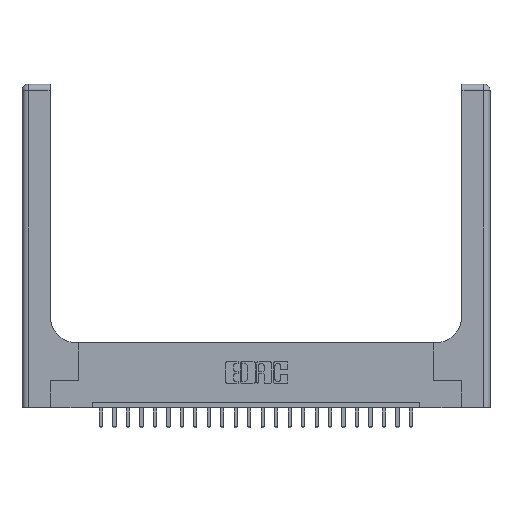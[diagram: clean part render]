
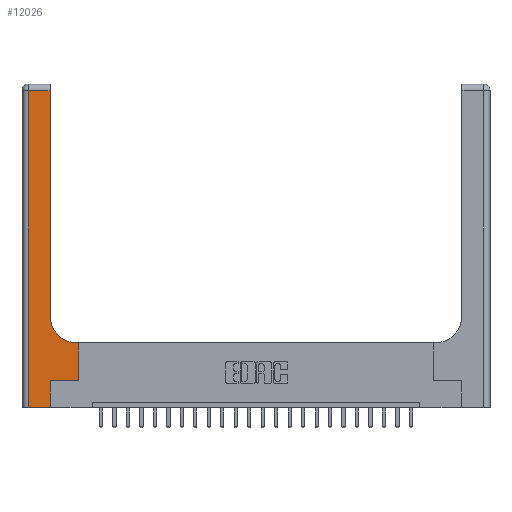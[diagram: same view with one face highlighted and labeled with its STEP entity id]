
A CAD part, top view. The second image highlights one B-rep face of the part: STEP entity #12026.
In plain terms, the highlighted planar face has unit normal (0, 0, 1).
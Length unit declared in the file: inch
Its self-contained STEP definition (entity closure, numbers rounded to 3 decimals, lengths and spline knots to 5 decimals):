
#301 = CARTESIAN_POINT ( 'NONE',  ( 0.528, 0.6, 0.37 ) ) ;
#339 = LINE ( 'NONE', #14077, #1956 ) ;
#576 = DIRECTION ( 'NONE',  ( 1., 0., 0. ) ) ;
#1641 = VECTOR ( 'NONE', #16301, 39.37008 ) ;
#1911 = CARTESIAN_POINT ( 'NONE',  ( 0.26, 3., 0.37 ) ) ;
#1956 = VECTOR ( 'NONE', #22181, 39.37008 ) ;
#2137 = ORIENTED_EDGE ( 'NONE', *, *, #9708, .T. ) ;
#2504 = EDGE_CURVE ( 'NONE', #5481, #12135, #12380, .T. ) ;
#2639 = DIRECTION ( 'NONE',  ( 1., 0., 0. ) ) ;
#2939 = CARTESIAN_POINT ( 'NONE',  ( 0.265, 0., 0.37 ) ) ;
#3023 = LINE ( 'NONE', #12256, #21039 ) ;
#3322 = ORIENTED_EDGE ( 'NONE', *, *, #9574, .T. ) ;
#3435 = CARTESIAN_POINT ( 'NONE',  ( 0.06, 3., 0.37 ) ) ;
#3584 = ORIENTED_EDGE ( 'NONE', *, *, #2504, .T. ) ;
#3600 = EDGE_CURVE ( 'NONE', #12812, #16042, #7360, .T. ) ;
#3667 = DIRECTION ( 'NONE',  ( 0., -1., 0. ) ) ;
#3821 = CARTESIAN_POINT ( 'NONE',  ( 0.06, 2.94, 0.37 ) ) ;
#3824 = FACE_OUTER_BOUND ( 'NONE', #8915, .T. ) ;
#4841 = ORIENTED_EDGE ( 'NONE', *, *, #3600, .T. ) ;
#5481 = VERTEX_POINT ( 'NONE', #21734 ) ;
#5776 = VECTOR ( 'NONE', #576, 39.37008 ) ;
#6133 = CIRCLE ( 'NONE', #20960, 0.25 ) ;
#7071 = CARTESIAN_POINT ( 'NONE',  ( 0.51, 0.6, 0.37 ) ) ;
#7234 = CARTESIAN_POINT ( 'NONE',  ( 0.26, 0.85, 0.37 ) ) ;
#7360 = LINE ( 'NONE', #17850, #18804 ) ;
#7581 = EDGE_CURVE ( 'NONE', #16042, #15617, #339, .T. ) ;
#7746 = VECTOR ( 'NONE', #2639, 39.37008 ) ;
#8087 = PLANE ( 'NONE',  #21438 ) ;
#8350 = CARTESIAN_POINT ( 'NONE',  ( 0.26, 2.94, 0.37 ) ) ;
#8547 = CARTESIAN_POINT ( 'NONE',  ( 0.265, 0.25, 0.37 ) ) ;
#8595 = VECTOR ( 'NONE', #14398, 39.37008 ) ;
#8769 = DIRECTION ( 'NONE',  ( 0., 0., -1. ) ) ;
#8854 = DIRECTION ( 'NONE',  ( 1., 0., 0. ) ) ;
#8915 = EDGE_LOOP ( 'NONE', ( #14490, #12352, #15742, #3584, #2137, #14130, #4841, #22571, #3322 ) ) ;
#9363 = DIRECTION ( 'NONE',  ( 0., 1., 0. ) ) ;
#9574 = EDGE_CURVE ( 'NONE', #15617, #15629, #6133, .T. ) ;
#9708 = EDGE_CURVE ( 'NONE', #12135, #17680, #10790, .T. ) ;
#10790 = LINE ( 'NONE', #17848, #8595 ) ;
#10931 = CARTESIAN_POINT ( 'NONE',  ( 0., 0., 0.37 ) ) ;
#10977 = LINE ( 'NONE', #1911, #1641 ) ;
#12026 = ADVANCED_FACE ( 'NONE', ( #3824 ), #8087, .F. ) ;
#12104 = CARTESIAN_POINT ( 'NONE',  ( 0.528, 0.25, 0.37 ) ) ;
#12135 = VERTEX_POINT ( 'NONE', #2939 ) ;
#12251 = VECTOR ( 'NONE', #3667, 39.37008 ) ;
#12256 = CARTESIAN_POINT ( 'NONE',  ( 0., 2.94, 0.37 ) ) ;
#12352 = ORIENTED_EDGE ( 'NONE', *, *, #18068, .T. ) ;
#12380 = LINE ( 'NONE', #10931, #5776 ) ;
#12812 = VERTEX_POINT ( 'NONE', #12104 ) ;
#12911 = EDGE_CURVE ( 'NONE', #14332, #5481, #22086, .T. ) ;
#14077 = CARTESIAN_POINT ( 'NONE',  ( 0.26, 0.6, 0.37 ) ) ;
#14130 = ORIENTED_EDGE ( 'NONE', *, *, #17398, .T. ) ;
#14332 = VERTEX_POINT ( 'NONE', #3821 ) ;
#14398 = DIRECTION ( 'NONE',  ( 0., 1., 0. ) ) ;
#14490 = ORIENTED_EDGE ( 'NONE', *, *, #19109, .T. ) ;
#15617 = VERTEX_POINT ( 'NONE', #7071 ) ;
#15629 = VERTEX_POINT ( 'NONE', #7234 ) ;
#15742 = ORIENTED_EDGE ( 'NONE', *, *, #12911, .T. ) ;
#16042 = VERTEX_POINT ( 'NONE', #301 ) ;
#16301 = DIRECTION ( 'NONE',  ( 0., 1., 0. ) ) ;
#16805 = CARTESIAN_POINT ( 'NONE',  ( 0.265, 0.25, 0.37 ) ) ;
#16902 = VERTEX_POINT ( 'NONE', #8350 ) ;
#17398 = EDGE_CURVE ( 'NONE', #17680, #12812, #18907, .T. ) ;
#17680 = VERTEX_POINT ( 'NONE', #8547 ) ;
#17848 = CARTESIAN_POINT ( 'NONE',  ( 0.265, 0., 0.37 ) ) ;
#17850 = CARTESIAN_POINT ( 'NONE',  ( 0.528, 0.25, 0.37 ) ) ;
#18068 = EDGE_CURVE ( 'NONE', #16902, #14332, #3023, .T. ) ;
#18804 = VECTOR ( 'NONE', #9363, 39.37008 ) ;
#18907 = LINE ( 'NONE', #16805, #7746 ) ;
#19109 = EDGE_CURVE ( 'NONE', #15629, #16902, #10977, .T. ) ;
#20044 = CARTESIAN_POINT ( 'NONE',  ( 0., 3., 0.37 ) ) ;
#20782 = DIRECTION ( 'NONE',  ( -1., 0., 0. ) ) ;
#20960 = AXIS2_PLACEMENT_3D ( 'NONE', #22550, #8769, #8854 ) ;
#21039 = VECTOR ( 'NONE', #20782, 39.37008 ) ;
#21438 = AXIS2_PLACEMENT_3D ( 'NONE', #20044, #21731, #22033 ) ;
#21731 = DIRECTION ( 'NONE',  ( 0., 0., -1. ) ) ;
#21734 = CARTESIAN_POINT ( 'NONE',  ( 0.06, 0., 0.37 ) ) ;
#22033 = DIRECTION ( 'NONE',  ( -1., 0., 0. ) ) ;
#22086 = LINE ( 'NONE', #3435, #12251 ) ;
#22181 = DIRECTION ( 'NONE',  ( -1., 0., 0. ) ) ;
#22550 = CARTESIAN_POINT ( 'NONE',  ( 0.51, 0.85, 0.37 ) ) ;
#22571 = ORIENTED_EDGE ( 'NONE', *, *, #7581, .T. ) ;
